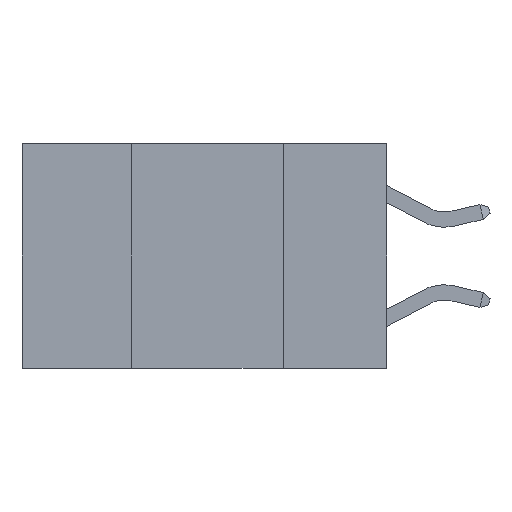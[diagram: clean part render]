
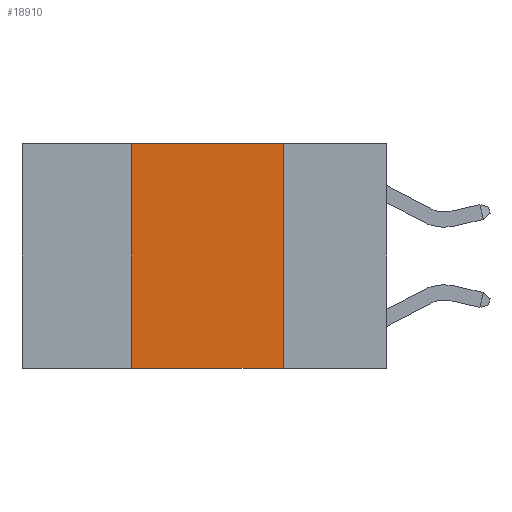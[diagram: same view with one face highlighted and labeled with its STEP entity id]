
A CAD part, left-side view. The second image highlights one B-rep face of the part: STEP entity #18910.
In plain terms, the highlighted planar face has unit normal (-1, 0, 0).
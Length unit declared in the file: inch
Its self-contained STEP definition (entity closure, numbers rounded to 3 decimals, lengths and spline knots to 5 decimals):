
#14 = VECTOR ( 'NONE', #1453, 39.37008 ) ;
#895 = PLANE ( 'NONE',  #9008 ) ;
#1453 = DIRECTION ( 'NONE',  ( 0., -1., 0. ) ) ;
#1563 = DIRECTION ( 'NONE',  ( 0., 0., 1. ) ) ;
#1817 = DIRECTION ( 'NONE',  ( 0., -1., 0. ) ) ;
#1853 = LINE ( 'NONE', #13759, #15967 ) ;
#1973 = LINE ( 'NONE', #3555, #6307 ) ;
#2110 = EDGE_CURVE ( 'NONE', #2777, #5598, #1853, .T. ) ;
#2273 = DIRECTION ( 'NONE',  ( 0., 0., -1. ) ) ;
#2631 = EDGE_CURVE ( 'NONE', #5598, #16559, #9309, .T. ) ;
#2777 = VERTEX_POINT ( 'NONE', #12453 ) ;
#3555 = CARTESIAN_POINT ( 'NONE',  ( 0., 0.17, 0. ) ) ;
#5449 = EDGE_CURVE ( 'NONE', #16559, #6558, #1973, .T. ) ;
#5530 = CARTESIAN_POINT ( 'NONE',  ( 0., 0.6, 0. ) ) ;
#5598 = VERTEX_POINT ( 'NONE', #6900 ) ;
#6307 = VECTOR ( 'NONE', #6320, 39.37008 ) ;
#6320 = DIRECTION ( 'NONE',  ( 0., 0., -1. ) ) ;
#6558 = VERTEX_POINT ( 'NONE', #16031 ) ;
#6900 = CARTESIAN_POINT ( 'NONE',  ( 0., 0.42, 0. ) ) ;
#6944 = ORIENTED_EDGE ( 'NONE', *, *, #16960, .T. ) ;
#7074 = ORIENTED_EDGE ( 'NONE', *, *, #5449, .F. ) ;
#8118 = CARTESIAN_POINT ( 'NONE',  ( 0., 0.6, -0.37 ) ) ;
#8318 = VECTOR ( 'NONE', #1817, 39.37008 ) ;
#8386 = FACE_OUTER_BOUND ( 'NONE', #11913, .T. ) ;
#8515 = CARTESIAN_POINT ( 'NONE',  ( 0., 0.17, 0. ) ) ;
#9008 = AXIS2_PLACEMENT_3D ( 'NONE', #5530, #11534, #2273 ) ;
#9309 = LINE ( 'NONE', #15307, #14 ) ;
#11534 = DIRECTION ( 'NONE',  ( 1., 0., 0. ) ) ;
#11913 = EDGE_LOOP ( 'NONE', ( #7074, #16307, #13213, #6944 ) ) ;
#12054 = LINE ( 'NONE', #8118, #8318 ) ;
#12453 = CARTESIAN_POINT ( 'NONE',  ( 0., 0.42, -0.37 ) ) ;
#13213 = ORIENTED_EDGE ( 'NONE', *, *, #2110, .F. ) ;
#13759 = CARTESIAN_POINT ( 'NONE',  ( 0., 0.42, 0. ) ) ;
#15307 = CARTESIAN_POINT ( 'NONE',  ( 0., 0.6, 0. ) ) ;
#15967 = VECTOR ( 'NONE', #1563, 39.37008 ) ;
#16031 = CARTESIAN_POINT ( 'NONE',  ( 0., 0.17, -0.37 ) ) ;
#16307 = ORIENTED_EDGE ( 'NONE', *, *, #2631, .F. ) ;
#16559 = VERTEX_POINT ( 'NONE', #8515 ) ;
#16960 = EDGE_CURVE ( 'NONE', #2777, #6558, #12054, .T. ) ;
#18910 = ADVANCED_FACE ( 'NONE', ( #8386 ), #895, .F. ) ;
